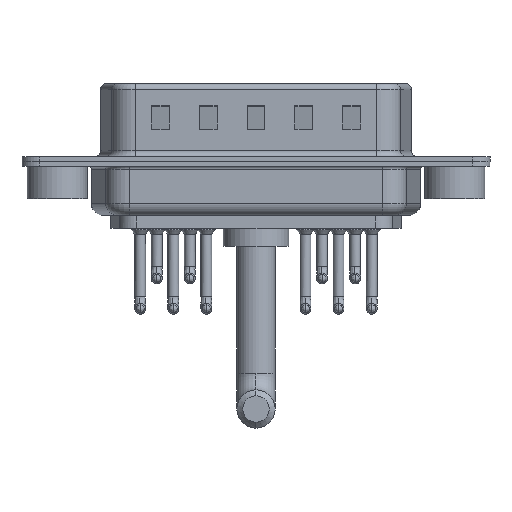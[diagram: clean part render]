
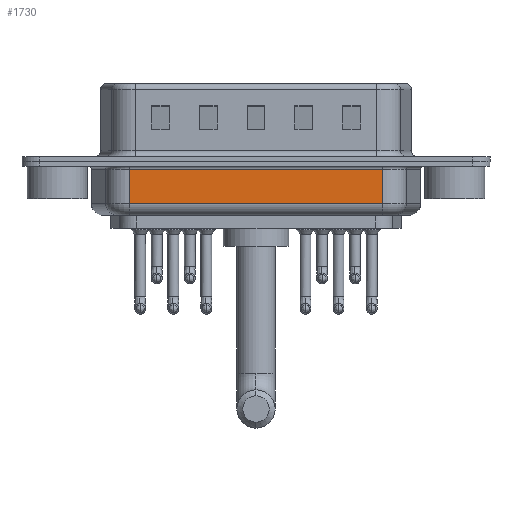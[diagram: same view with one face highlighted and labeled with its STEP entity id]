
A CAD part, front view. The second image highlights one B-rep face of the part: STEP entity #1730.
In plain terms, the highlighted planar face has unit normal (0, -1, 0).
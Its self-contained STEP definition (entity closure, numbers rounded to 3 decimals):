
#537 = EDGE_CURVE ( 'NONE', #12845, #7990, #10595, .T. ) ;
#653 = VECTOR ( 'NONE', #6742, 1000. ) ;
#976 = LINE ( 'NONE', #21720, #19523 ) ;
#1104 = CARTESIAN_POINT ( 'NONE',  ( 6.031, -5.35, -3.5 ) ) ;
#1730 = ADVANCED_FACE ( 'NONE', ( #17067 ), #15580, .F. ) ;
#2259 = VECTOR ( 'NONE', #8801, 1000. ) ;
#2353 = VERTEX_POINT ( 'NONE', #4555 ) ;
#3324 = ORIENTED_EDGE ( 'NONE', *, *, #15829, .T. ) ;
#3339 = CARTESIAN_POINT ( 'NONE',  ( 6.031, -5.35, -4.5 ) ) ;
#4555 = CARTESIAN_POINT ( 'NONE',  ( 27.269, -5.35, -0.65 ) ) ;
#4966 = VECTOR ( 'NONE', #9322, 1000. ) ;
#6742 = DIRECTION ( 'NONE',  ( 0., 0., 1. ) ) ;
#7990 = VERTEX_POINT ( 'NONE', #17385 ) ;
#8348 = DIRECTION ( 'NONE',  ( 0., 0., 1. ) ) ;
#8801 = DIRECTION ( 'NONE',  ( 1., 0., 0. ) ) ;
#8837 = ORIENTED_EDGE ( 'NONE', *, *, #18242, .T. ) ;
#9077 = CARTESIAN_POINT ( 'NONE',  ( 6.031, -5.35, -0.65 ) ) ;
#9322 = DIRECTION ( 'NONE',  ( -1., 0., 0. ) ) ;
#9809 = DIRECTION ( 'NONE',  ( 0., 0., 1. ) ) ;
#10262 = DIRECTION ( 'NONE',  ( 0., 1., 0. ) ) ;
#10595 = LINE ( 'NONE', #13887, #2259 ) ;
#10752 = ORIENTED_EDGE ( 'NONE', *, *, #537, .T. ) ;
#10864 = ORIENTED_EDGE ( 'NONE', *, *, #15279, .F. ) ;
#11013 = AXIS2_PLACEMENT_3D ( 'NONE', #3339, #10262, #8348 ) ;
#11539 = VERTEX_POINT ( 'NONE', #9077 ) ;
#12845 = VERTEX_POINT ( 'NONE', #1104 ) ;
#13887 = CARTESIAN_POINT ( 'NONE',  ( 6.031, -5.35, -3.5 ) ) ;
#15047 = EDGE_LOOP ( 'NONE', ( #10864, #10752, #8837, #3324 ) ) ;
#15279 = EDGE_CURVE ( 'NONE', #12845, #11539, #15353, .T. ) ;
#15353 = LINE ( 'NONE', #20560, #653 ) ;
#15580 = PLANE ( 'NONE',  #11013 ) ;
#15829 = EDGE_CURVE ( 'NONE', #2353, #11539, #17703, .T. ) ;
#17067 = FACE_OUTER_BOUND ( 'NONE', #15047, .T. ) ;
#17385 = CARTESIAN_POINT ( 'NONE',  ( 27.269, -5.35, -3.5 ) ) ;
#17703 = LINE ( 'NONE', #17928, #4966 ) ;
#17928 = CARTESIAN_POINT ( 'NONE',  ( 6.031, -5.35, -0.65 ) ) ;
#18242 = EDGE_CURVE ( 'NONE', #7990, #2353, #976, .T. ) ;
#19523 = VECTOR ( 'NONE', #9809, 1000. ) ;
#20560 = CARTESIAN_POINT ( 'NONE',  ( 6.031, -5.35, -4.5 ) ) ;
#21720 = CARTESIAN_POINT ( 'NONE',  ( 27.269, -5.35, -4.5 ) ) ;
